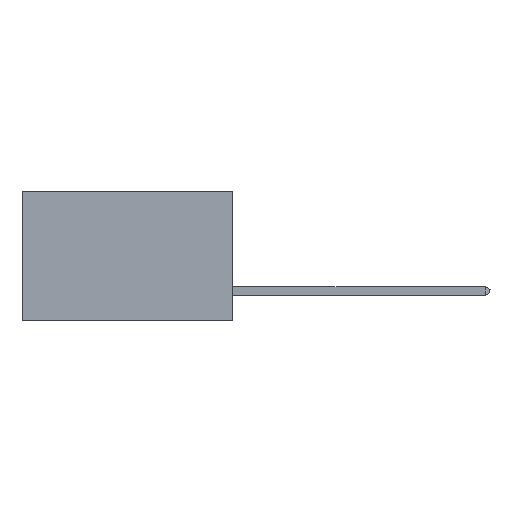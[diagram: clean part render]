
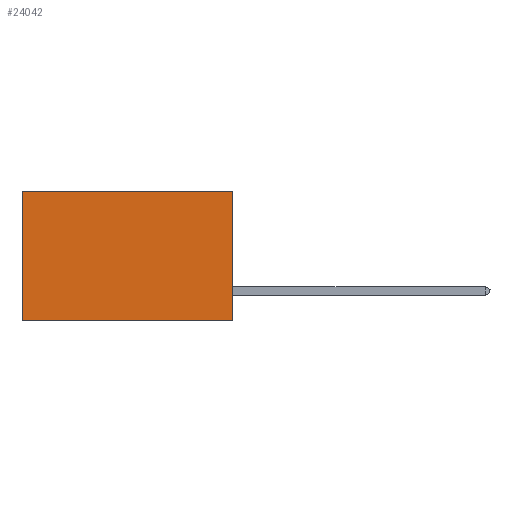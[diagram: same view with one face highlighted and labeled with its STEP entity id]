
A CAD part, left-side view. The second image highlights one B-rep face of the part: STEP entity #24042.
In plain terms, the highlighted planar face has unit normal (-1, 0, 0).
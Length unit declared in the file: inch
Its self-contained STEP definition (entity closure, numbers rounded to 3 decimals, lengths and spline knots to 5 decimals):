
#14 = EDGE_CURVE ( 'NONE', #12438, #30289, #20250, .T. ) ;
#984 = AXIS2_PLACEMENT_3D ( 'NONE', #22721, #4734, #10825 ) ;
#4734 = DIRECTION ( 'NONE',  ( 1., 0., 0. ) ) ;
#6209 = DIRECTION ( 'NONE',  ( 0., 0., -1. ) ) ;
#6496 = DIRECTION ( 'NONE',  ( 0., 0., -1. ) ) ;
#6658 = VECTOR ( 'NONE', #6209, 39.37008 ) ;
#8990 = CARTESIAN_POINT ( 'NONE',  ( 0.2875, 0.6, 0. ) ) ;
#9563 = CARTESIAN_POINT ( 'NONE',  ( 0.2875, 0., 0. ) ) ;
#10162 = LINE ( 'NONE', #26106, #20563 ) ;
#10825 = DIRECTION ( 'NONE',  ( 0., 0., -1. ) ) ;
#12337 = VERTEX_POINT ( 'NONE', #24192 ) ;
#12438 = VERTEX_POINT ( 'NONE', #9563 ) ;
#14266 = DIRECTION ( 'NONE',  ( 0., 1., 0. ) ) ;
#14891 = EDGE_CURVE ( 'NONE', #30289, #12337, #23062, .T. ) ;
#15121 = VERTEX_POINT ( 'NONE', #8990 ) ;
#16717 = PLANE ( 'NONE',  #984 ) ;
#17315 = EDGE_LOOP ( 'NONE', ( #33651, #21632, #30217, #37683 ) ) ;
#17361 = CARTESIAN_POINT ( 'NONE',  ( 0.2875, 0., -0.37 ) ) ;
#20250 = LINE ( 'NONE', #27295, #6658 ) ;
#20563 = VECTOR ( 'NONE', #6496, 39.37008 ) ;
#21213 = VECTOR ( 'NONE', #35160, 39.37008 ) ;
#21632 = ORIENTED_EDGE ( 'NONE', *, *, #14891, .F. ) ;
#22721 = CARTESIAN_POINT ( 'NONE',  ( 0.2875, 0., 0. ) ) ;
#23062 = LINE ( 'NONE', #17361, #21213 ) ;
#24042 = ADVANCED_FACE ( 'NONE', ( #34926 ), #16717, .F. ) ;
#24192 = CARTESIAN_POINT ( 'NONE',  ( 0.2875, 0.6, -0.37 ) ) ;
#24375 = EDGE_CURVE ( 'NONE', #15121, #12337, #10162, .T. ) ;
#25531 = CARTESIAN_POINT ( 'NONE',  ( 0.2875, 0., -0.37 ) ) ;
#25879 = VECTOR ( 'NONE', #14266, 39.37008 ) ;
#26106 = CARTESIAN_POINT ( 'NONE',  ( 0.2875, 0.6, 0. ) ) ;
#26299 = CARTESIAN_POINT ( 'NONE',  ( 0.2875, 0., 0. ) ) ;
#27295 = CARTESIAN_POINT ( 'NONE',  ( 0.2875, 0., 0. ) ) ;
#27735 = LINE ( 'NONE', #26299, #25879 ) ;
#30217 = ORIENTED_EDGE ( 'NONE', *, *, #14, .F. ) ;
#30289 = VERTEX_POINT ( 'NONE', #25531 ) ;
#33651 = ORIENTED_EDGE ( 'NONE', *, *, #24375, .T. ) ;
#34926 = FACE_OUTER_BOUND ( 'NONE', #17315, .T. ) ;
#35045 = EDGE_CURVE ( 'NONE', #12438, #15121, #27735, .T. ) ;
#35160 = DIRECTION ( 'NONE',  ( 0., 1., 0. ) ) ;
#37683 = ORIENTED_EDGE ( 'NONE', *, *, #35045, .T. ) ;
